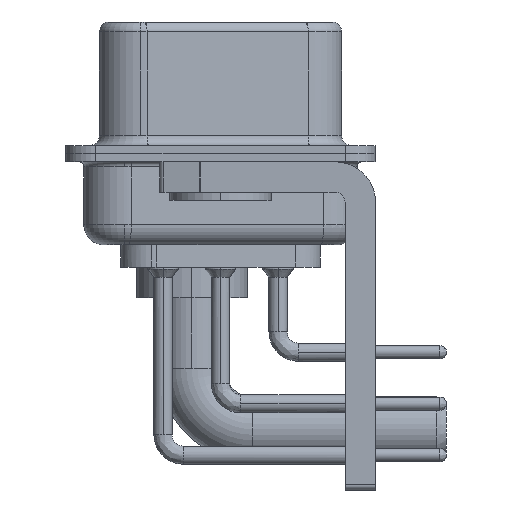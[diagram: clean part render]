
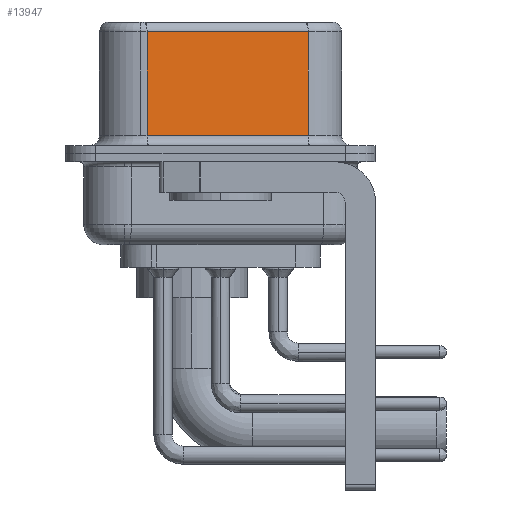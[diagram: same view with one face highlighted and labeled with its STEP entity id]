
A CAD part, left-side view. The second image highlights one B-rep face of the part: STEP entity #13947.
In plain terms, the highlighted planar face has unit normal (-0.985, -0.174, 0).
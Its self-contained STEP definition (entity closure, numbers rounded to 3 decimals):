
#2338 = VERTEX_POINT ( 'NONE', #21399 ) ;
#3956 = DIRECTION ( 'NONE',  ( -0.174, 0.985, 0. ) ) ;
#4746 = CARTESIAN_POINT ( 'NONE',  ( 5.132, -4.322, 0.9 ) ) ;
#5028 = VECTOR ( 'NONE', #20857, 1000. ) ;
#6836 = CARTESIAN_POINT ( 'NONE',  ( 5.132, -4.322, 6.52 ) ) ;
#7033 = DIRECTION ( 'NONE',  ( 0.985, 0.174, 0. ) ) ;
#7687 = CARTESIAN_POINT ( 'NONE',  ( 5.132, -4.322, 6.52 ) ) ;
#8109 = VERTEX_POINT ( 'NONE', #4746 ) ;
#8822 = EDGE_CURVE ( 'NONE', #30106, #2338, #9129, .T. ) ;
#9129 = LINE ( 'NONE', #31883, #5028 ) ;
#9409 = CARTESIAN_POINT ( 'NONE',  ( 5.132, -4.322, 6.02 ) ) ;
#10539 = VERTEX_POINT ( 'NONE', #9409 ) ;
#13329 = ORIENTED_EDGE ( 'NONE', *, *, #19884, .T. ) ;
#13947 = ADVANCED_FACE ( 'NONE', ( #15159 ), #33475, .F. ) ;
#14779 = ORIENTED_EDGE ( 'NONE', *, *, #8822, .T. ) ;
#15159 = FACE_OUTER_BOUND ( 'NONE', #29454, .T. ) ;
#16432 = ORIENTED_EDGE ( 'NONE', *, *, #22803, .T. ) ;
#18600 = DIRECTION ( 'NONE',  ( -0.174, 0.985, 0. ) ) ;
#18824 = LINE ( 'NONE', #30399, #27615 ) ;
#19884 = EDGE_CURVE ( 'NONE', #2338, #8109, #24886, .T. ) ;
#20437 = EDGE_CURVE ( 'NONE', #10539, #8109, #25235, .T. ) ;
#20711 = AXIS2_PLACEMENT_3D ( 'NONE', #6836, #7033, #18600 ) ;
#20857 = DIRECTION ( 'NONE',  ( 0., 0., -1. ) ) ;
#21399 = CARTESIAN_POINT ( 'NONE',  ( 3.73, 3.628, 0.9 ) ) ;
#22190 = CARTESIAN_POINT ( 'NONE',  ( 5.132, -4.322, 0.9 ) ) ;
#22417 = ORIENTED_EDGE ( 'NONE', *, *, #20437, .F. ) ;
#22803 = EDGE_CURVE ( 'NONE', #10539, #30106, #18824, .T. ) ;
#24886 = LINE ( 'NONE', #22190, #26175 ) ;
#25235 = LINE ( 'NONE', #7687, #25628 ) ;
#25628 = VECTOR ( 'NONE', #31776, 1000. ) ;
#26175 = VECTOR ( 'NONE', #36493, 1000. ) ;
#27615 = VECTOR ( 'NONE', #3956, 1000. ) ;
#28459 = CARTESIAN_POINT ( 'NONE',  ( 3.73, 3.628, 6.02 ) ) ;
#29454 = EDGE_LOOP ( 'NONE', ( #22417, #16432, #14779, #13329 ) ) ;
#30106 = VERTEX_POINT ( 'NONE', #28459 ) ;
#30399 = CARTESIAN_POINT ( 'NONE',  ( 5.132, -4.322, 6.02 ) ) ;
#31776 = DIRECTION ( 'NONE',  ( 0., 0., -1. ) ) ;
#31883 = CARTESIAN_POINT ( 'NONE',  ( 3.73, 3.628, 6.52 ) ) ;
#33475 = PLANE ( 'NONE',  #20711 ) ;
#36493 = DIRECTION ( 'NONE',  ( 0.174, -0.985, 0. ) ) ;
